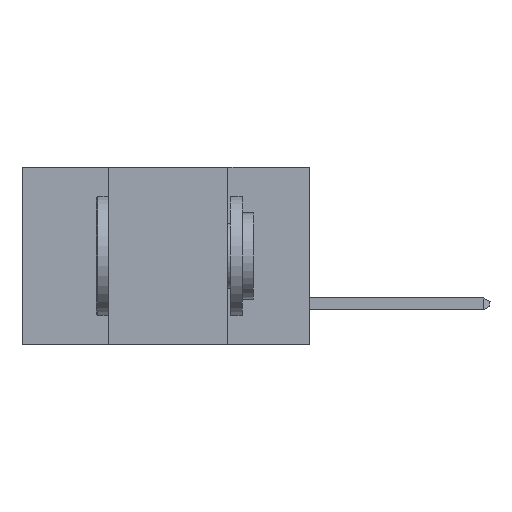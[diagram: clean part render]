
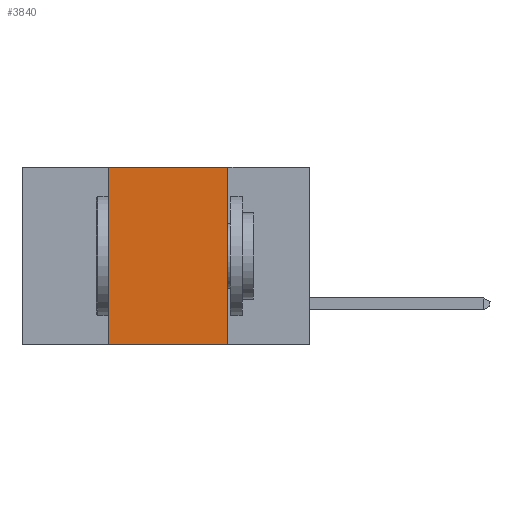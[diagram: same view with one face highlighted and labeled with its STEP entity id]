
A CAD part, left-side view. The second image highlights one B-rep face of the part: STEP entity #3840.
In plain terms, the highlighted planar face has unit normal (-1, 0, 0).
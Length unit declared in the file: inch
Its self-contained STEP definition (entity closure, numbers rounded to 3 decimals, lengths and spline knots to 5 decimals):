
#1503 = CARTESIAN_POINT ( 'NONE',  ( 0., 0.17, 0. ) ) ;
#3486 = VERTEX_POINT ( 'NONE', #6446 ) ;
#3840 = ADVANCED_FACE ( 'NONE', ( #33689 ), #27812, .F. ) ;
#3857 = EDGE_CURVE ( 'NONE', #3486, #22477, #5407, .T. ) ;
#4676 = CARTESIAN_POINT ( 'NONE',  ( 0., 0.6, 0. ) ) ;
#4725 = VECTOR ( 'NONE', #42952, 39.37008 ) ;
#5407 = LINE ( 'NONE', #15170, #30037 ) ;
#5865 = LINE ( 'NONE', #37812, #42152 ) ;
#6446 = CARTESIAN_POINT ( 'NONE',  ( 0., 0.42, -0.37 ) ) ;
#7908 = LINE ( 'NONE', #13319, #4725 ) ;
#13319 = CARTESIAN_POINT ( 'NONE',  ( 0., 0.6, 0. ) ) ;
#15170 = CARTESIAN_POINT ( 'NONE',  ( 0., 0.6, -0.37 ) ) ;
#19643 = CARTESIAN_POINT ( 'NONE',  ( 0., 0.42, 0. ) ) ;
#21147 = VECTOR ( 'NONE', #31554, 39.37008 ) ;
#21546 = CARTESIAN_POINT ( 'NONE',  ( 0., 0.17, 0. ) ) ;
#22477 = VERTEX_POINT ( 'NONE', #38467 ) ;
#24488 = DIRECTION ( 'NONE',  ( 0., 0., 1. ) ) ;
#24930 = DIRECTION ( 'NONE',  ( 1., 0., 0. ) ) ;
#26669 = ORIENTED_EDGE ( 'NONE', *, *, #3857, .T. ) ;
#27364 = EDGE_LOOP ( 'NONE', ( #31513, #41440, #29354, #26669 ) ) ;
#27812 = PLANE ( 'NONE',  #42658 ) ;
#27956 = DIRECTION ( 'NONE',  ( 0., -1., 0. ) ) ;
#28890 = EDGE_CURVE ( 'NONE', #28915, #22477, #35776, .T. ) ;
#28915 = VERTEX_POINT ( 'NONE', #21546 ) ;
#29354 = ORIENTED_EDGE ( 'NONE', *, *, #32980, .F. ) ;
#29799 = EDGE_CURVE ( 'NONE', #33933, #28915, #7908, .T. ) ;
#30037 = VECTOR ( 'NONE', #27956, 39.37008 ) ;
#31513 = ORIENTED_EDGE ( 'NONE', *, *, #28890, .F. ) ;
#31554 = DIRECTION ( 'NONE',  ( 0., 0., -1. ) ) ;
#32980 = EDGE_CURVE ( 'NONE', #3486, #33933, #5865, .T. ) ;
#33689 = FACE_OUTER_BOUND ( 'NONE', #27364, .T. ) ;
#33933 = VERTEX_POINT ( 'NONE', #19643 ) ;
#35776 = LINE ( 'NONE', #1503, #21147 ) ;
#37812 = CARTESIAN_POINT ( 'NONE',  ( 0., 0.42, 0. ) ) ;
#38467 = CARTESIAN_POINT ( 'NONE',  ( 0., 0.17, -0.37 ) ) ;
#38563 = DIRECTION ( 'NONE',  ( 0., 0., -1. ) ) ;
#41440 = ORIENTED_EDGE ( 'NONE', *, *, #29799, .F. ) ;
#42152 = VECTOR ( 'NONE', #24488, 39.37008 ) ;
#42658 = AXIS2_PLACEMENT_3D ( 'NONE', #4676, #24930, #38563 ) ;
#42952 = DIRECTION ( 'NONE',  ( 0., -1., 0. ) ) ;
